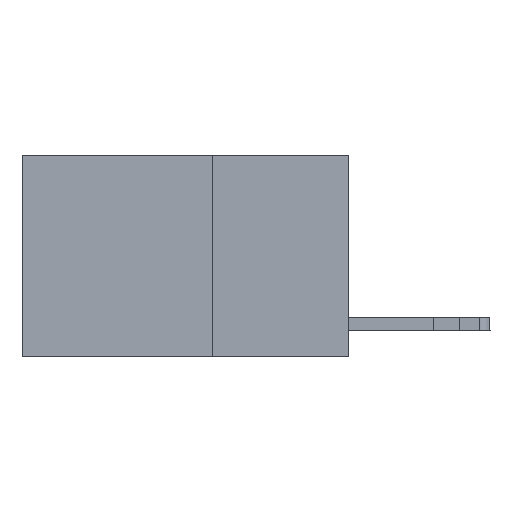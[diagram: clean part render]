
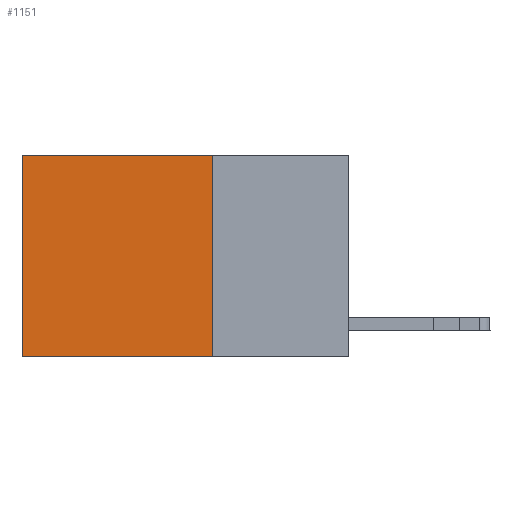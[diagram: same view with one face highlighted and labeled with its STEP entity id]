
A CAD part, left-side view. The second image highlights one B-rep face of the part: STEP entity #1151.
In plain terms, the highlighted planar face has unit normal (-1, 0, 0).
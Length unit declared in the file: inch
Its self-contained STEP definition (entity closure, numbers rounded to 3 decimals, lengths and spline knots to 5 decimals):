
#260 = CARTESIAN_POINT ( 'NONE',  ( 0.2625, 0.25, -0.37 ) ) ;
#328 = LINE ( 'NONE', #17061, #5838 ) ;
#576 = VERTEX_POINT ( 'NONE', #13643 ) ;
#1151 = ADVANCED_FACE ( 'NONE', ( #5124 ), #19728, .F. ) ;
#1477 = ORIENTED_EDGE ( 'NONE', *, *, #4247, .F. ) ;
#3035 = CARTESIAN_POINT ( 'NONE',  ( 0.2625, 0.25, 0. ) ) ;
#3229 = LINE ( 'NONE', #6974, #7303 ) ;
#3795 = CARTESIAN_POINT ( 'NONE',  ( 0.2625, 0.25, -0.37 ) ) ;
#4247 = EDGE_CURVE ( 'NONE', #22860, #576, #23969, .T. ) ;
#4515 = LINE ( 'NONE', #21418, #7399 ) ;
#5124 = FACE_OUTER_BOUND ( 'NONE', #9104, .T. ) ;
#5838 = VECTOR ( 'NONE', #15086, 39.37008 ) ;
#5883 = VERTEX_POINT ( 'NONE', #14928 ) ;
#6974 = CARTESIAN_POINT ( 'NONE',  ( 0.2625, 0.6, 0. ) ) ;
#7303 = VECTOR ( 'NONE', #14413, 39.37008 ) ;
#7399 = VECTOR ( 'NONE', #15335, 39.37008 ) ;
#9104 = EDGE_LOOP ( 'NONE', ( #17141, #1477, #20443, #21367 ) ) ;
#9398 = CARTESIAN_POINT ( 'NONE',  ( 0.2625, 0.6, 0. ) ) ;
#10788 = AXIS2_PLACEMENT_3D ( 'NONE', #3035, #12521, #15816 ) ;
#11838 = EDGE_CURVE ( 'NONE', #15222, #576, #3229, .T. ) ;
#12446 = EDGE_CURVE ( 'NONE', #5883, #22860, #328, .T. ) ;
#12521 = DIRECTION ( 'NONE',  ( 1., 0., 0. ) ) ;
#12608 = EDGE_CURVE ( 'NONE', #5883, #15222, #4515, .T. ) ;
#13025 = DIRECTION ( 'NONE',  ( 0., 1., 0. ) ) ;
#13643 = CARTESIAN_POINT ( 'NONE',  ( 0.2625, 0.6, -0.37 ) ) ;
#14413 = DIRECTION ( 'NONE',  ( 0., 0., -1. ) ) ;
#14928 = CARTESIAN_POINT ( 'NONE',  ( 0.2625, 0.25, 0. ) ) ;
#15086 = DIRECTION ( 'NONE',  ( 0., 0., -1. ) ) ;
#15222 = VERTEX_POINT ( 'NONE', #9398 ) ;
#15335 = DIRECTION ( 'NONE',  ( 0., 1., 0. ) ) ;
#15816 = DIRECTION ( 'NONE',  ( 0., 0., -1. ) ) ;
#17061 = CARTESIAN_POINT ( 'NONE',  ( 0.2625, 0.25, 0. ) ) ;
#17141 = ORIENTED_EDGE ( 'NONE', *, *, #11838, .T. ) ;
#18735 = VECTOR ( 'NONE', #13025, 39.37008 ) ;
#19728 = PLANE ( 'NONE',  #10788 ) ;
#20443 = ORIENTED_EDGE ( 'NONE', *, *, #12446, .F. ) ;
#21367 = ORIENTED_EDGE ( 'NONE', *, *, #12608, .T. ) ;
#21418 = CARTESIAN_POINT ( 'NONE',  ( 0.2625, 0.25, 0. ) ) ;
#22860 = VERTEX_POINT ( 'NONE', #260 ) ;
#23969 = LINE ( 'NONE', #3795, #18735 ) ;
